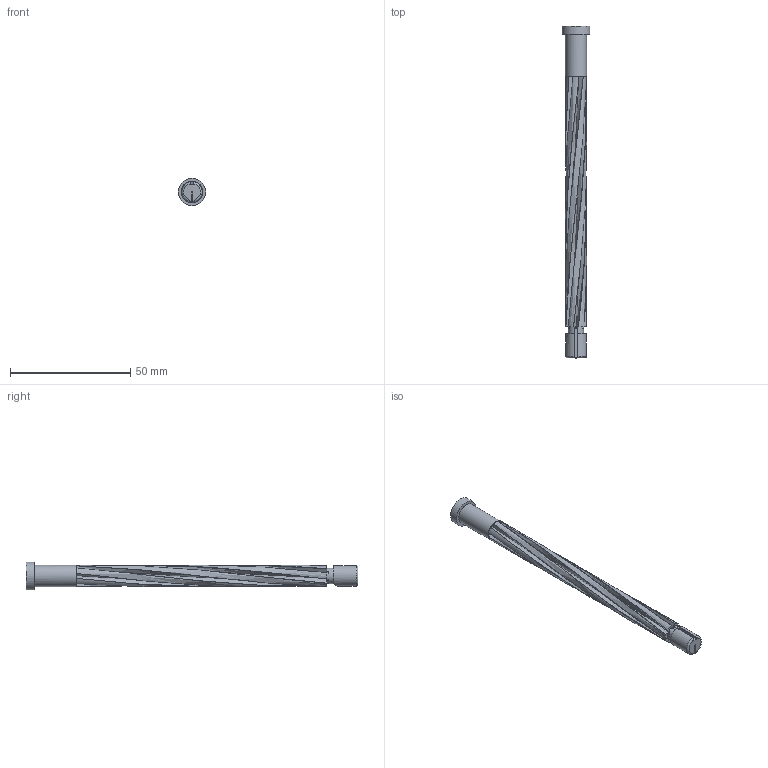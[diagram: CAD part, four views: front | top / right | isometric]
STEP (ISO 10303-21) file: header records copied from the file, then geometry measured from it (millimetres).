
FILE_DESCRIPTION(/* description */ (''),/* implementation_level */ '2;1');
FILE_NAME(/* name */ 'Rifling Mandrel-9x19-6gr-polygonal-1in9.82-Twist-8.82mm-Bore.stp',/* time_stamp */ '2019-12-05T11:04:50-06:00',/* author */ ('johne'),/* organization */ (''),/* preprocessor_version */ 'ST-DEVELOPER v18',/* originating_system */ 'Autodesk Inventor 2020',/* authorisation */ '');
FILE_SCHEMA (('AUTOMOTIVE_DESIGN { 1 0 10303 214 3 1 1 }'));
Length unit declared in the file: inch
Products named in the file (1): Rifling Mandrel
Bounding box: 11.46 x 137.84 x 11.46 mm (x, y, z)
Volume: 6704.8 mm3; surface area: 6454.6 mm2
Topology: 1 solids, 1 shells, 181 faces, 564 edges, 380 vertices
Faces by surface type: bspline 103, plane 32, cylinder 31, torus 8, cone 6, sphere 1
Full cylindrical faces by diameter (mm): 8.82 x1, 11.464 x1
Entity records: 9317 total; most frequent: CARTESIAN_POINT 5297, ORIENTED_EDGE 1126, EDGE_CURVE 563, B_SPLINE_CURVE_WITH_KNOTS 423, VERTEX_POINT 380, DIRECTION 380, EDGE_LOOP 189, FACE_OUTER_BOUND 181
